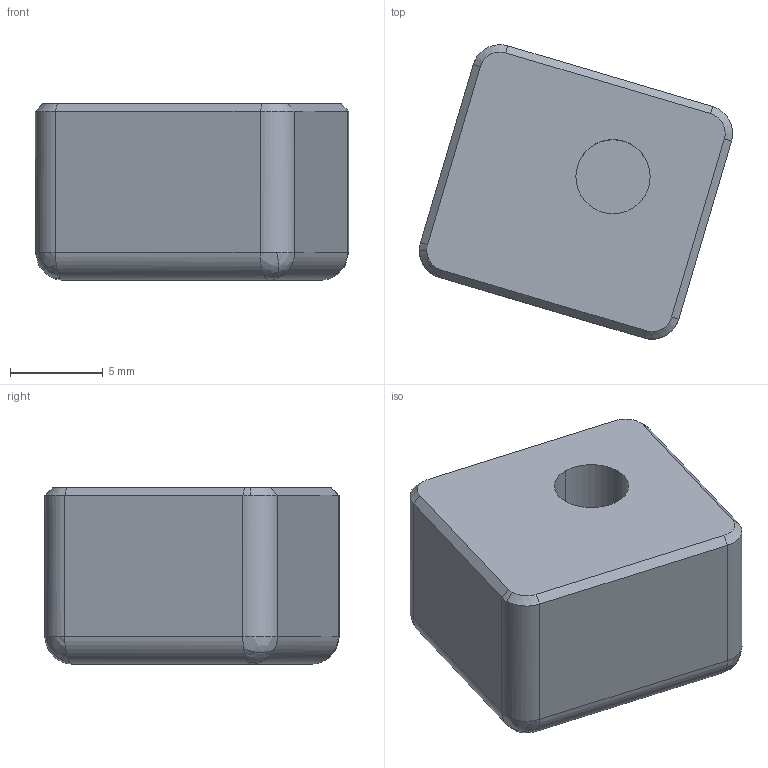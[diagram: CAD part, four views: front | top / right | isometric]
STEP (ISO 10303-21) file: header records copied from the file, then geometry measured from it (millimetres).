
FILE_DESCRIPTION (( 'STEP AP203' ), '1' );
FILE_NAME ('MOD9_V3_Mag_Release_Button.STEP', '2020-12-23T19:07:35', ( '' ), ( '' ), 'SwSTEP 2.0', 'SolidWorks 2019', '' );
FILE_SCHEMA (( 'CONFIG_CONTROL_DESIGN' ));
Length unit declared in the file: millimetre
Products named in the file (1): MOD9_V3_Mag_Release_Button
Bounding box: 16.87 x 15.85 x 9.5 mm (x, y, z)
Volume: 1668.6 mm3; surface area: 899.3 mm2
Topology: 1 solids, 1 shells, 35 faces, 88 edges, 48 vertices
Faces by surface type: cylinder 11, plane 11, bspline 8, cone 5
Entity records: 1152 total; most frequent: CARTESIAN_POINT 287, DIRECTION 177, ORIENTED_EDGE 160, EDGE_CURVE 80, AXIS2_PLACEMENT_3D 72, VERTEX_POINT 48, CIRCLE 44, EDGE_LOOP 36
